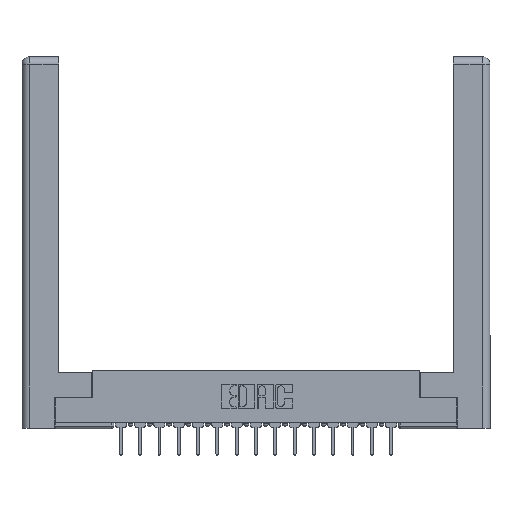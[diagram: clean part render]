
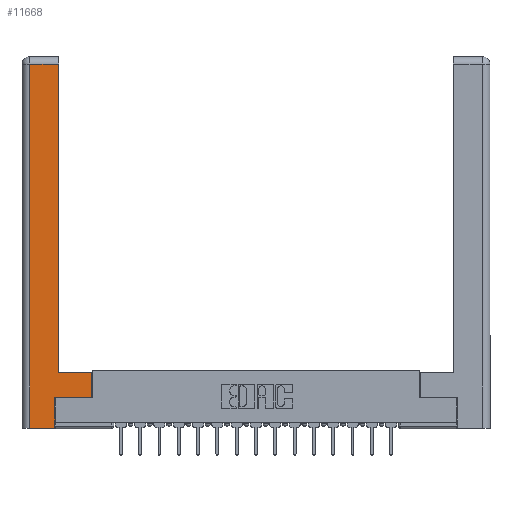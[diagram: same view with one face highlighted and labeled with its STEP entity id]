
A CAD part, top view. The second image highlights one B-rep face of the part: STEP entity #11668.
In plain terms, the highlighted planar face has unit normal (0, 0, 1).
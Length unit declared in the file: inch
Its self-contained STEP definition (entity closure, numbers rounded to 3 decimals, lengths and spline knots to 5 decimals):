
#117 = ORIENTED_EDGE ( 'NONE', *, *, #4579, .T. ) ;
#515 = VERTEX_POINT ( 'NONE', #13277 ) ;
#665 = LINE ( 'NONE', #18153, #11836 ) ;
#1000 = EDGE_CURVE ( 'NONE', #7692, #10860, #11541, .T. ) ;
#1173 = FACE_OUTER_BOUND ( 'NONE', #13294, .T. ) ;
#1527 = VECTOR ( 'NONE', #15312, 39.37008 ) ;
#1787 = VECTOR ( 'NONE', #15763, 39.37008 ) ;
#2006 = DIRECTION ( 'NONE',  ( 0., 1., 0. ) ) ;
#2300 = CARTESIAN_POINT ( 'NONE',  ( 0.295, 3., 0. ) ) ;
#3296 = DIRECTION ( 'NONE',  ( -1., 0., 0. ) ) ;
#3317 = CARTESIAN_POINT ( 'NONE',  ( 0.0615, 2.94, 0. ) ) ;
#3512 = VERTEX_POINT ( 'NONE', #17118 ) ;
#3608 = VERTEX_POINT ( 'NONE', #11523 ) ;
#3959 = ORIENTED_EDGE ( 'NONE', *, *, #16549, .T. ) ;
#4579 = EDGE_CURVE ( 'NONE', #515, #7692, #18080, .T. ) ;
#4690 = EDGE_CURVE ( 'NONE', #12770, #18028, #16884, .T. ) ;
#4717 = EDGE_CURVE ( 'NONE', #3512, #12770, #9235, .T. ) ;
#5279 = VECTOR ( 'NONE', #6574, 39.37008 ) ;
#5557 = ORIENTED_EDGE ( 'NONE', *, *, #9027, .T. ) ;
#6131 = EDGE_CURVE ( 'NONE', #18028, #3608, #8701, .T. ) ;
#6395 = CARTESIAN_POINT ( 'NONE',  ( 0.565, 0.45, 0. ) ) ;
#6574 = DIRECTION ( 'NONE',  ( 0., 1., 0. ) ) ;
#6852 = AXIS2_PLACEMENT_3D ( 'NONE', #9255, #18057, #3296 ) ;
#6928 = EDGE_CURVE ( 'NONE', #3608, #18631, #8430, .T. ) ;
#7508 = CARTESIAN_POINT ( 'NONE',  ( 0.565, 0.45, 0. ) ) ;
#7692 = VERTEX_POINT ( 'NONE', #13288 ) ;
#8055 = CARTESIAN_POINT ( 'NONE',  ( 0.295, 0.45, 0. ) ) ;
#8430 = LINE ( 'NONE', #3317, #11715 ) ;
#8701 = LINE ( 'NONE', #2300, #14745 ) ;
#8979 = VECTOR ( 'NONE', #13972, 39.37008 ) ;
#9027 = EDGE_CURVE ( 'NONE', #18631, #515, #18297, .T. ) ;
#9117 = PLANE ( 'NONE',  #6852 ) ;
#9235 = LINE ( 'NONE', #6395, #5279 ) ;
#9255 = CARTESIAN_POINT ( 'NONE',  ( 0., 0., 0. ) ) ;
#9437 = ORIENTED_EDGE ( 'NONE', *, *, #6928, .T. ) ;
#9466 = VECTOR ( 'NONE', #2006, 39.37008 ) ;
#10860 = VERTEX_POINT ( 'NONE', #17559 ) ;
#11328 = CARTESIAN_POINT ( 'NONE',  ( 0.265, 0., 0. ) ) ;
#11523 = CARTESIAN_POINT ( 'NONE',  ( 0.295, 2.94, 0. ) ) ;
#11541 = LINE ( 'NONE', #16211, #9466 ) ;
#11668 = ADVANCED_FACE ( 'NONE', ( #1173 ), #9117, .F. ) ;
#11715 = VECTOR ( 'NONE', #15825, 39.37008 ) ;
#11836 = VECTOR ( 'NONE', #17064, 39.37008 ) ;
#12770 = VERTEX_POINT ( 'NONE', #7508 ) ;
#12915 = CARTESIAN_POINT ( 'NONE',  ( 0.295, 0.45, 0. ) ) ;
#13243 = CARTESIAN_POINT ( 'NONE',  ( 0.0615, 2.94, 0. ) ) ;
#13277 = CARTESIAN_POINT ( 'NONE',  ( 0.0615, 0., 0. ) ) ;
#13288 = CARTESIAN_POINT ( 'NONE',  ( 0.265, 0., 0. ) ) ;
#13294 = EDGE_LOOP ( 'NONE', ( #13479, #9437, #5557, #117, #18916, #3959, #14911, #15404 ) ) ;
#13479 = ORIENTED_EDGE ( 'NONE', *, *, #6131, .T. ) ;
#13972 = DIRECTION ( 'NONE',  ( -1., 0., 0. ) ) ;
#14745 = VECTOR ( 'NONE', #15664, 39.37008 ) ;
#14911 = ORIENTED_EDGE ( 'NONE', *, *, #4717, .T. ) ;
#15312 = DIRECTION ( 'NONE',  ( 0., -1., 0. ) ) ;
#15404 = ORIENTED_EDGE ( 'NONE', *, *, #4690, .T. ) ;
#15664 = DIRECTION ( 'NONE',  ( 0., 1., 0. ) ) ;
#15763 = DIRECTION ( 'NONE',  ( 1., 0., 0. ) ) ;
#15825 = DIRECTION ( 'NONE',  ( -1., 0., 0. ) ) ;
#16211 = CARTESIAN_POINT ( 'NONE',  ( 0.265, 0.245, 0. ) ) ;
#16549 = EDGE_CURVE ( 'NONE', #10860, #3512, #665, .T. ) ;
#16884 = LINE ( 'NONE', #8055, #8979 ) ;
#17064 = DIRECTION ( 'NONE',  ( 1., 0., 0. ) ) ;
#17118 = CARTESIAN_POINT ( 'NONE',  ( 0.565, 0.245, 0. ) ) ;
#17559 = CARTESIAN_POINT ( 'NONE',  ( 0.265, 0.245, 0. ) ) ;
#18028 = VERTEX_POINT ( 'NONE', #12915 ) ;
#18057 = DIRECTION ( 'NONE',  ( 0., 0., -1. ) ) ;
#18080 = LINE ( 'NONE', #11328, #1787 ) ;
#18153 = CARTESIAN_POINT ( 'NONE',  ( 0.565, 0.245, 0. ) ) ;
#18297 = LINE ( 'NONE', #18324, #1527 ) ;
#18324 = CARTESIAN_POINT ( 'NONE',  ( 0.0615, 0., 0. ) ) ;
#18631 = VERTEX_POINT ( 'NONE', #13243 ) ;
#18916 = ORIENTED_EDGE ( 'NONE', *, *, #1000, .T. ) ;
